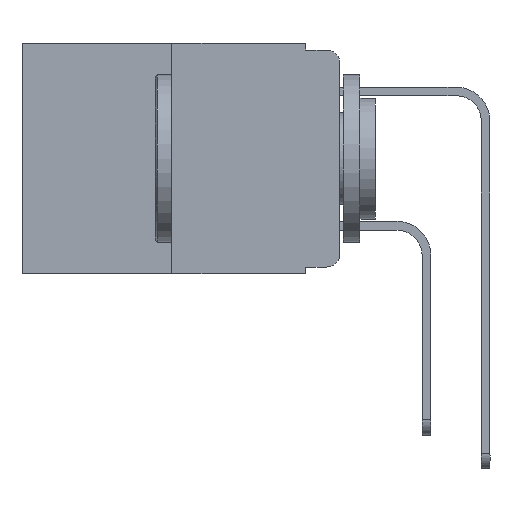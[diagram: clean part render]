
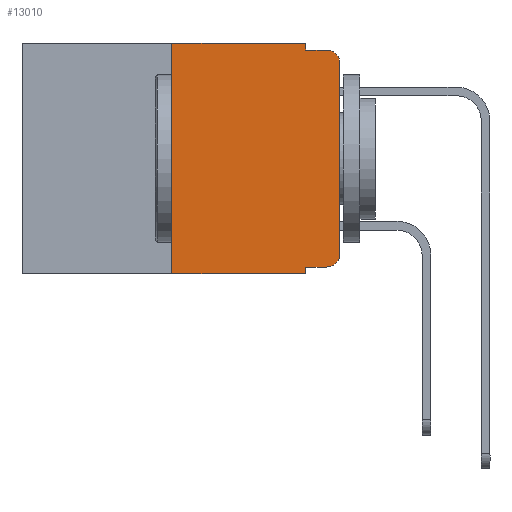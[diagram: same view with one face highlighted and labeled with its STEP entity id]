
A CAD part, left-side view. The second image highlights one B-rep face of the part: STEP entity #13010.
In plain terms, the highlighted planar face has unit normal (-1, 0, 0).
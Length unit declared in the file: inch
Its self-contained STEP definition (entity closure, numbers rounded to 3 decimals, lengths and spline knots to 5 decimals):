
#88 = DIRECTION ( 'NONE',  ( 0., 0., 1. ) ) ;
#92 = ORIENTED_EDGE ( 'NONE', *, *, #646, .F. ) ;
#105 = CARTESIAN_POINT ( 'NONE',  ( 0., 0.02, -0.333 ) ) ;
#116 = DIRECTION ( 'NONE',  ( 0., 0., -1. ) ) ;
#170 = CARTESIAN_POINT ( 'NONE',  ( 0., 0.25, -0.343 ) ) ;
#187 = LINE ( 'NONE', #13638, #12729 ) ;
#477 = AXIS2_PLACEMENT_3D ( 'NONE', #7608, #1001, #7838 ) ;
#588 = ORIENTED_EDGE ( 'NONE', *, *, #12926, .T. ) ;
#646 = EDGE_CURVE ( 'NONE', #10795, #8086, #2653, .T. ) ;
#660 = CIRCLE ( 'NONE', #3807, 0.02 ) ;
#761 = VECTOR ( 'NONE', #1520, 39.37008 ) ;
#1001 = DIRECTION ( 'NONE',  ( 1., 0., 0. ) ) ;
#1256 = ORIENTED_EDGE ( 'NONE', *, *, #4835, .F. ) ;
#1373 = VERTEX_POINT ( 'NONE', #13082 ) ;
#1520 = DIRECTION ( 'NONE',  ( 0., 0., -1. ) ) ;
#1812 = DIRECTION ( 'NONE',  ( 0., 0., -1. ) ) ;
#1857 = ORIENTED_EDGE ( 'NONE', *, *, #7720, .T. ) ;
#1891 = AXIS2_PLACEMENT_3D ( 'NONE', #8944, #11274, #12378 ) ;
#1913 = VERTEX_POINT ( 'NONE', #8280 ) ;
#2486 = EDGE_LOOP ( 'NONE', ( #12406, #2696, #7811, #4876, #1256, #13075, #1857, #92, #8549, #588 ) ) ;
#2527 = VERTEX_POINT ( 'NONE', #3436 ) ;
#2555 = VERTEX_POINT ( 'NONE', #6705 ) ;
#2653 = LINE ( 'NONE', #7162, #761 ) ;
#2696 = ORIENTED_EDGE ( 'NONE', *, *, #11589, .T. ) ;
#2809 = EDGE_CURVE ( 'NONE', #13632, #2527, #9811, .T. ) ;
#2915 = CARTESIAN_POINT ( 'NONE',  ( 0., 0.051, -0.333 ) ) ;
#2935 = CARTESIAN_POINT ( 'NONE',  ( 0., 0.02, -0.03 ) ) ;
#3002 = EDGE_CURVE ( 'NONE', #2555, #13632, #187, .T. ) ;
#3159 = PLANE ( 'NONE',  #477 ) ;
#3386 = VERTEX_POINT ( 'NONE', #7594 ) ;
#3436 = CARTESIAN_POINT ( 'NONE',  ( 0., 0.02, -0.01 ) ) ;
#3743 = CARTESIAN_POINT ( 'NONE',  ( 0., 0.473, 0. ) ) ;
#3807 = AXIS2_PLACEMENT_3D ( 'NONE', #2935, #13945, #1812 ) ;
#3928 = DIRECTION ( 'NONE',  ( 0., -1., 0. ) ) ;
#4005 = CARTESIAN_POINT ( 'NONE',  ( 0., 0.051, -0.343 ) ) ;
#4781 = VERTEX_POINT ( 'NONE', #170 ) ;
#4835 = EDGE_CURVE ( 'NONE', #1373, #2555, #6050, .T. ) ;
#4876 = ORIENTED_EDGE ( 'NONE', *, *, #3002, .F. ) ;
#4981 = VECTOR ( 'NONE', #14188, 39.37008 ) ;
#5934 = VECTOR ( 'NONE', #13844, 39.37008 ) ;
#6050 = LINE ( 'NONE', #3743, #5934 ) ;
#6419 = EDGE_CURVE ( 'NONE', #4781, #1373, #10086, .T. ) ;
#6705 = CARTESIAN_POINT ( 'NONE',  ( 0., 0.051, 0. ) ) ;
#6805 = VECTOR ( 'NONE', #12826, 39.37008 ) ;
#7091 = LINE ( 'NONE', #11573, #6805 ) ;
#7162 = CARTESIAN_POINT ( 'NONE',  ( 0., 0.051, 0. ) ) ;
#7594 = CARTESIAN_POINT ( 'NONE',  ( 0., 0., -0.313 ) ) ;
#7608 = CARTESIAN_POINT ( 'NONE',  ( 0., 0.473, 0. ) ) ;
#7720 = EDGE_CURVE ( 'NONE', #4781, #8086, #7091, .T. ) ;
#7769 = VECTOR ( 'NONE', #11942, 39.37008 ) ;
#7811 = ORIENTED_EDGE ( 'NONE', *, *, #2809, .F. ) ;
#7838 = DIRECTION ( 'NONE',  ( 0., 0., -1. ) ) ;
#8086 = VERTEX_POINT ( 'NONE', #4005 ) ;
#8280 = CARTESIAN_POINT ( 'NONE',  ( 0., 0., -0.03 ) ) ;
#8295 = CIRCLE ( 'NONE', #1891, 0.02 ) ;
#8518 = VECTOR ( 'NONE', #3928, 39.37008 ) ;
#8549 = ORIENTED_EDGE ( 'NONE', *, *, #11101, .T. ) ;
#8719 = FACE_OUTER_BOUND ( 'NONE', #2486, .T. ) ;
#8872 = CARTESIAN_POINT ( 'NONE',  ( 0., 0.051, -0.01 ) ) ;
#8944 = CARTESIAN_POINT ( 'NONE',  ( 0., 0.02, -0.313 ) ) ;
#9348 = VERTEX_POINT ( 'NONE', #105 ) ;
#9811 = LINE ( 'NONE', #8872, #7769 ) ;
#10086 = LINE ( 'NONE', #11181, #10288 ) ;
#10288 = VECTOR ( 'NONE', #88, 39.37008 ) ;
#10795 = VERTEX_POINT ( 'NONE', #2915 ) ;
#10876 = CARTESIAN_POINT ( 'NONE',  ( 0., 0., 0. ) ) ;
#11101 = EDGE_CURVE ( 'NONE', #10795, #9348, #13884, .T. ) ;
#11181 = CARTESIAN_POINT ( 'NONE',  ( 0., 0.25, 0. ) ) ;
#11274 = DIRECTION ( 'NONE',  ( -1., 0., 0. ) ) ;
#11573 = CARTESIAN_POINT ( 'NONE',  ( 0., 0.473, -0.343 ) ) ;
#11589 = EDGE_CURVE ( 'NONE', #1913, #2527, #660, .T. ) ;
#11942 = DIRECTION ( 'NONE',  ( 0., -1., 0. ) ) ;
#12378 = DIRECTION ( 'NONE',  ( 0., 0., -1. ) ) ;
#12406 = ORIENTED_EDGE ( 'NONE', *, *, #12572, .T. ) ;
#12432 = CARTESIAN_POINT ( 'NONE',  ( 0., 0.051, -0.01 ) ) ;
#12572 = EDGE_CURVE ( 'NONE', #3386, #1913, #13240, .T. ) ;
#12729 = VECTOR ( 'NONE', #116, 39.37008 ) ;
#12826 = DIRECTION ( 'NONE',  ( 0., -1., 0. ) ) ;
#12926 = EDGE_CURVE ( 'NONE', #9348, #3386, #8295, .T. ) ;
#13010 = ADVANCED_FACE ( 'NONE', ( #8719 ), #3159, .F. ) ;
#13075 = ORIENTED_EDGE ( 'NONE', *, *, #6419, .F. ) ;
#13079 = CARTESIAN_POINT ( 'NONE',  ( 0., 0.051, -0.333 ) ) ;
#13082 = CARTESIAN_POINT ( 'NONE',  ( 0., 0.25, 0. ) ) ;
#13240 = LINE ( 'NONE', #10876, #4981 ) ;
#13632 = VERTEX_POINT ( 'NONE', #12432 ) ;
#13638 = CARTESIAN_POINT ( 'NONE',  ( 0., 0.051, 0. ) ) ;
#13844 = DIRECTION ( 'NONE',  ( 0., -1., 0. ) ) ;
#13884 = LINE ( 'NONE', #13079, #8518 ) ;
#13945 = DIRECTION ( 'NONE',  ( -1., 0., 0. ) ) ;
#14188 = DIRECTION ( 'NONE',  ( 0., 0., 1. ) ) ;
